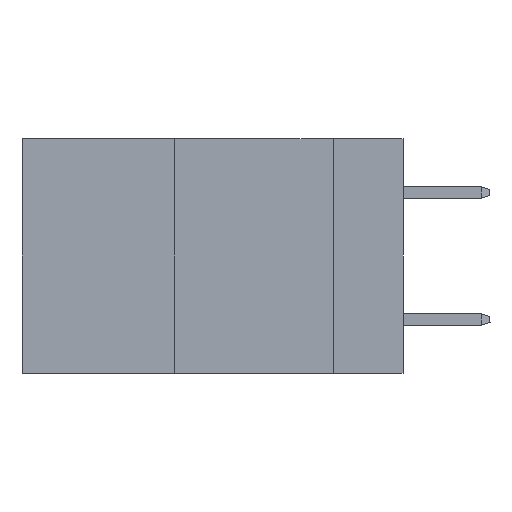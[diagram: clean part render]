
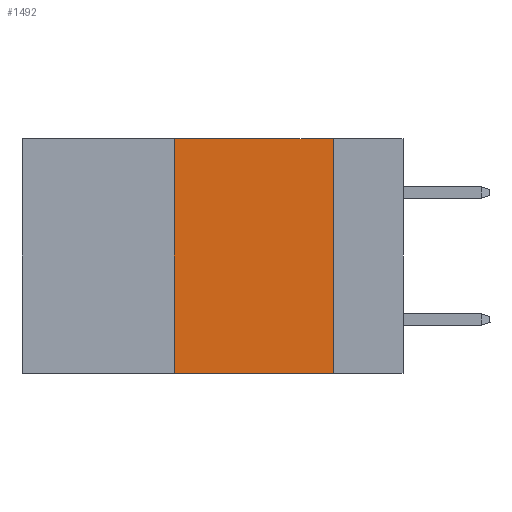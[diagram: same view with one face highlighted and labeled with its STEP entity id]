
A CAD part, left-side view. The second image highlights one B-rep face of the part: STEP entity #1492.
In plain terms, the highlighted planar face has unit normal (-1, 0, 0).
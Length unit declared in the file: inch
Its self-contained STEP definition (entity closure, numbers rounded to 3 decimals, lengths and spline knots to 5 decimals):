
#197 = PLANE ( 'NONE',  #12927 ) ;
#353 = VECTOR ( 'NONE', #10088, 39.37008 ) ;
#1034 = DIRECTION ( 'NONE',  ( 0., 0., -1. ) ) ;
#1122 = DIRECTION ( 'NONE',  ( 0., 0., -1. ) ) ;
#1492 = ADVANCED_FACE ( 'NONE', ( #13380 ), #197, .F. ) ;
#2099 = LINE ( 'NONE', #12940, #7176 ) ;
#2567 = CARTESIAN_POINT ( 'NONE',  ( 0., 0.11, -0.37 ) ) ;
#2580 = DIRECTION ( 'NONE',  ( 0., -1., 0. ) ) ;
#4139 = EDGE_LOOP ( 'NONE', ( #5841, #16389, #6922, #4152 ) ) ;
#4152 = ORIENTED_EDGE ( 'NONE', *, *, #13349, .T. ) ;
#4293 = VECTOR ( 'NONE', #8498, 39.37008 ) ;
#4466 = DIRECTION ( 'NONE',  ( 1., 0., 0. ) ) ;
#4648 = VERTEX_POINT ( 'NONE', #6094 ) ;
#5295 = CARTESIAN_POINT ( 'NONE',  ( 0., 0.6, 0. ) ) ;
#5841 = ORIENTED_EDGE ( 'NONE', *, *, #13423, .F. ) ;
#6094 = CARTESIAN_POINT ( 'NONE',  ( 0., 0.36, -0.37 ) ) ;
#6327 = VECTOR ( 'NONE', #2580, 39.37008 ) ;
#6360 = CARTESIAN_POINT ( 'NONE',  ( 0., 0.6, -0.37 ) ) ;
#6897 = CARTESIAN_POINT ( 'NONE',  ( 0., 0.11, 0. ) ) ;
#6922 = ORIENTED_EDGE ( 'NONE', *, *, #12691, .F. ) ;
#7163 = LINE ( 'NONE', #11251, #4293 ) ;
#7176 = VECTOR ( 'NONE', #1034, 39.37008 ) ;
#7622 = EDGE_CURVE ( 'NONE', #8516, #16639, #17504, .T. ) ;
#8498 = DIRECTION ( 'NONE',  ( 0., 0., 1. ) ) ;
#8516 = VERTEX_POINT ( 'NONE', #9411 ) ;
#9411 = CARTESIAN_POINT ( 'NONE',  ( 0., 0.36, 0. ) ) ;
#9463 = VERTEX_POINT ( 'NONE', #2567 ) ;
#10088 = DIRECTION ( 'NONE',  ( 0., -1., 0. ) ) ;
#11251 = CARTESIAN_POINT ( 'NONE',  ( 0., 0.36, 0. ) ) ;
#12691 = EDGE_CURVE ( 'NONE', #4648, #8516, #7163, .T. ) ;
#12927 = AXIS2_PLACEMENT_3D ( 'NONE', #5295, #4466, #1122 ) ;
#12940 = CARTESIAN_POINT ( 'NONE',  ( 0., 0.11, 0. ) ) ;
#13349 = EDGE_CURVE ( 'NONE', #4648, #9463, #14187, .T. ) ;
#13380 = FACE_OUTER_BOUND ( 'NONE', #4139, .T. ) ;
#13423 = EDGE_CURVE ( 'NONE', #16639, #9463, #2099, .T. ) ;
#14187 = LINE ( 'NONE', #6360, #353 ) ;
#16097 = CARTESIAN_POINT ( 'NONE',  ( 0., 0.6, 0. ) ) ;
#16389 = ORIENTED_EDGE ( 'NONE', *, *, #7622, .F. ) ;
#16639 = VERTEX_POINT ( 'NONE', #6897 ) ;
#17504 = LINE ( 'NONE', #16097, #6327 ) ;
